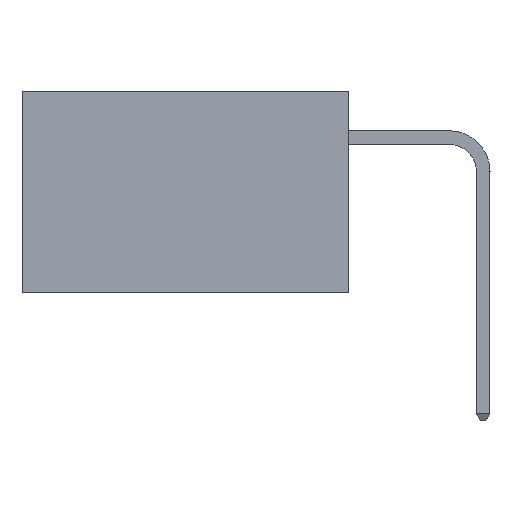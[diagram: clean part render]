
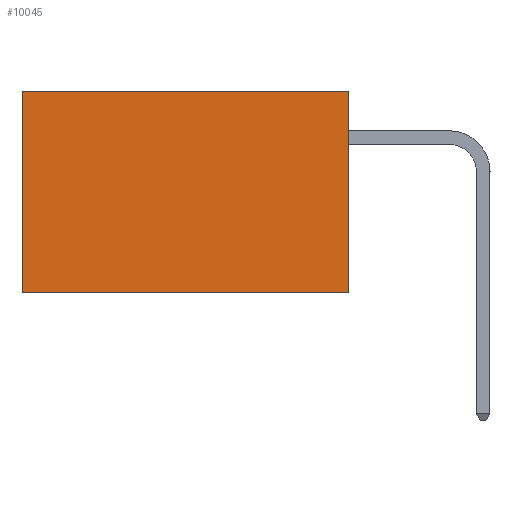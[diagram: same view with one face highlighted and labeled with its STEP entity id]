
A CAD part, left-side view. The second image highlights one B-rep face of the part: STEP entity #10045.
In plain terms, the highlighted planar face has unit normal (-1, 0, 0).
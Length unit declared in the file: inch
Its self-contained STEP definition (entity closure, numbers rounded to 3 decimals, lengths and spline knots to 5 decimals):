
#499 = DIRECTION ( 'NONE',  ( 1., 0., 0. ) ) ;
#1165 = VECTOR ( 'NONE', #18008, 39.37008 ) ;
#1224 = VECTOR ( 'NONE', #3086, 39.37008 ) ;
#1766 = VERTEX_POINT ( 'NONE', #4520 ) ;
#2015 = DIRECTION ( 'NONE',  ( 0., 0., -1. ) ) ;
#2221 = FACE_OUTER_BOUND ( 'NONE', #11716, .T. ) ;
#2365 = VECTOR ( 'NONE', #14614, 39.37008 ) ;
#3086 = DIRECTION ( 'NONE',  ( 0., 1., 0. ) ) ;
#4520 = CARTESIAN_POINT ( 'NONE',  ( 0.2875, 0.6, -0.37 ) ) ;
#4970 = AXIS2_PLACEMENT_3D ( 'NONE', #17284, #499, #11317 ) ;
#5094 = EDGE_CURVE ( 'NONE', #10758, #1766, #17476, .T. ) ;
#5510 = CARTESIAN_POINT ( 'NONE',  ( 0.2875, 0., 0. ) ) ;
#6923 = CARTESIAN_POINT ( 'NONE',  ( 0.2875, 0., -0.37 ) ) ;
#6961 = ORIENTED_EDGE ( 'NONE', *, *, #5094, .F. ) ;
#7091 = EDGE_CURVE ( 'NONE', #10410, #1766, #12710, .T. ) ;
#7870 = EDGE_CURVE ( 'NONE', #12725, #10758, #18465, .T. ) ;
#8999 = LINE ( 'NONE', #13539, #1165 ) ;
#9850 = PLANE ( 'NONE',  #4970 ) ;
#10045 = ADVANCED_FACE ( 'NONE', ( #2221 ), #9850, .F. ) ;
#10148 = CARTESIAN_POINT ( 'NONE',  ( 0.2875, 0., -0.37 ) ) ;
#10410 = VERTEX_POINT ( 'NONE', #15167 ) ;
#10758 = VERTEX_POINT ( 'NONE', #6923 ) ;
#10786 = ORIENTED_EDGE ( 'NONE', *, *, #7870, .F. ) ;
#10893 = EDGE_CURVE ( 'NONE', #12725, #10410, #8999, .T. ) ;
#11317 = DIRECTION ( 'NONE',  ( 0., 0., -1. ) ) ;
#11716 = EDGE_LOOP ( 'NONE', ( #17152, #6961, #10786, #17463 ) ) ;
#12710 = LINE ( 'NONE', #18646, #17157 ) ;
#12725 = VERTEX_POINT ( 'NONE', #18999 ) ;
#13539 = CARTESIAN_POINT ( 'NONE',  ( 0.2875, 0., 0. ) ) ;
#14614 = DIRECTION ( 'NONE',  ( 0., 0., -1. ) ) ;
#15167 = CARTESIAN_POINT ( 'NONE',  ( 0.2875, 0.6, 0. ) ) ;
#17152 = ORIENTED_EDGE ( 'NONE', *, *, #7091, .T. ) ;
#17157 = VECTOR ( 'NONE', #2015, 39.37008 ) ;
#17284 = CARTESIAN_POINT ( 'NONE',  ( 0.2875, 0., 0. ) ) ;
#17463 = ORIENTED_EDGE ( 'NONE', *, *, #10893, .T. ) ;
#17476 = LINE ( 'NONE', #10148, #1224 ) ;
#18008 = DIRECTION ( 'NONE',  ( 0., 1., 0. ) ) ;
#18465 = LINE ( 'NONE', #5510, #2365 ) ;
#18646 = CARTESIAN_POINT ( 'NONE',  ( 0.2875, 0.6, 0. ) ) ;
#18999 = CARTESIAN_POINT ( 'NONE',  ( 0.2875, 0., 0. ) ) ;
